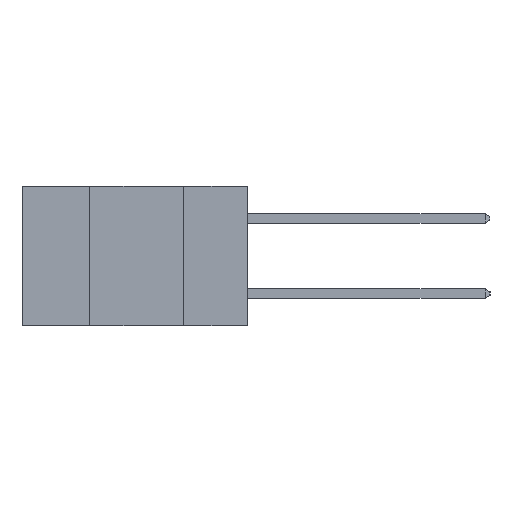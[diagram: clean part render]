
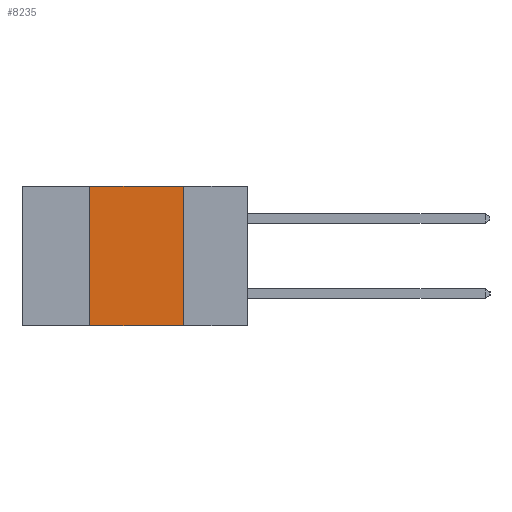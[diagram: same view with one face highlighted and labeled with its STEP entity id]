
A CAD part, left-side view. The second image highlights one B-rep face of the part: STEP entity #8235.
In plain terms, the highlighted planar face has unit normal (-1, 0, 0).
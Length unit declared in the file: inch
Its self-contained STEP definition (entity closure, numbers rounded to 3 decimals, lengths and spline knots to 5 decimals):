
#331 = VERTEX_POINT ( 'NONE', #7212 ) ;
#805 = AXIS2_PLACEMENT_3D ( 'NONE', #9176, #9997, #4942 ) ;
#1006 = CARTESIAN_POINT ( 'NONE',  ( 0., 0.17, -0.37 ) ) ;
#1441 = CARTESIAN_POINT ( 'NONE',  ( 0., 0.6, -0.37 ) ) ;
#1629 = ORIENTED_EDGE ( 'NONE', *, *, #5558, .F. ) ;
#1819 = CARTESIAN_POINT ( 'NONE',  ( 0., 0.17, 0. ) ) ;
#1842 = LINE ( 'NONE', #1441, #3781 ) ;
#2392 = CARTESIAN_POINT ( 'NONE',  ( 0., 0.42, -0.37 ) ) ;
#2486 = EDGE_LOOP ( 'NONE', ( #3118, #9315, #1629, #3704 ) ) ;
#3080 = VERTEX_POINT ( 'NONE', #1819 ) ;
#3118 = ORIENTED_EDGE ( 'NONE', *, *, #7109, .F. ) ;
#3278 = PLANE ( 'NONE',  #805 ) ;
#3328 = EDGE_CURVE ( 'NONE', #7484, #3851, #1842, .T. ) ;
#3367 = LINE ( 'NONE', #9077, #8378 ) ;
#3704 = ORIENTED_EDGE ( 'NONE', *, *, #3328, .T. ) ;
#3781 = VECTOR ( 'NONE', #5757, 39.37008 ) ;
#3851 = VERTEX_POINT ( 'NONE', #10560 ) ;
#3991 = DIRECTION ( 'NONE',  ( 0., 0., 1. ) ) ;
#4213 = VECTOR ( 'NONE', #7733, 39.37008 ) ;
#4496 = VECTOR ( 'NONE', #8064, 39.37008 ) ;
#4942 = DIRECTION ( 'NONE',  ( 0., 0., -1. ) ) ;
#5558 = EDGE_CURVE ( 'NONE', #7484, #331, #3367, .T. ) ;
#5757 = DIRECTION ( 'NONE',  ( 0., -1., 0. ) ) ;
#6143 = EDGE_CURVE ( 'NONE', #331, #3080, #9022, .T. ) ;
#6867 = FACE_OUTER_BOUND ( 'NONE', #2486, .T. ) ;
#7109 = EDGE_CURVE ( 'NONE', #3080, #3851, #8728, .T. ) ;
#7212 = CARTESIAN_POINT ( 'NONE',  ( 0., 0.42, 0. ) ) ;
#7230 = CARTESIAN_POINT ( 'NONE',  ( 0., 0.6, 0. ) ) ;
#7484 = VERTEX_POINT ( 'NONE', #2392 ) ;
#7733 = DIRECTION ( 'NONE',  ( 0., 0., -1. ) ) ;
#8064 = DIRECTION ( 'NONE',  ( 0., -1., 0. ) ) ;
#8235 = ADVANCED_FACE ( 'NONE', ( #6867 ), #3278, .F. ) ;
#8378 = VECTOR ( 'NONE', #3991, 39.37008 ) ;
#8728 = LINE ( 'NONE', #1006, #4213 ) ;
#9022 = LINE ( 'NONE', #7230, #4496 ) ;
#9077 = CARTESIAN_POINT ( 'NONE',  ( 0., 0.42, -0.37 ) ) ;
#9176 = CARTESIAN_POINT ( 'NONE',  ( 0., 0.6, 0. ) ) ;
#9315 = ORIENTED_EDGE ( 'NONE', *, *, #6143, .F. ) ;
#9997 = DIRECTION ( 'NONE',  ( 1., 0., 0. ) ) ;
#10560 = CARTESIAN_POINT ( 'NONE',  ( 0., 0.17, -0.37 ) ) ;
